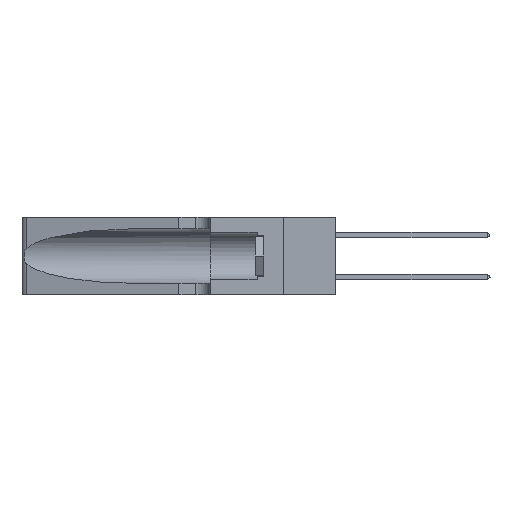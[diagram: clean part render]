
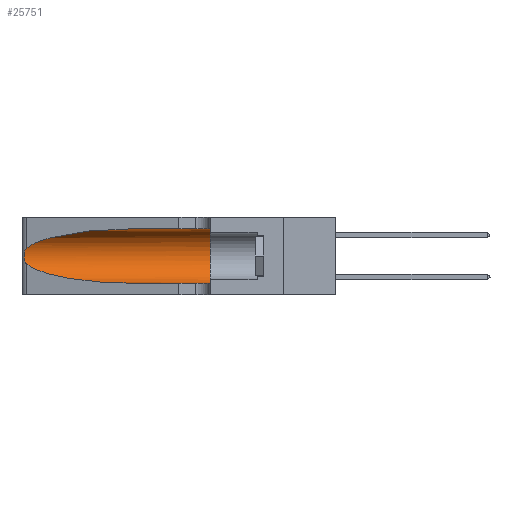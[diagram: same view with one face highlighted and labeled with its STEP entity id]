
A CAD part, left-side view. The second image highlights one B-rep face of the part: STEP entity #25751.
In plain terms, the highlighted cylindrical face has radius 3.308 mm (diameter 6.617 mm), a partial arc.
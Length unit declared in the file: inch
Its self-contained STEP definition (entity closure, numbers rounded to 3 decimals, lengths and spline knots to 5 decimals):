
#13 = EDGE_CURVE ( 'NONE', #23263, #21131, #15037, .T. ) ;
#1695 = CARTESIAN_POINT ( 'NONE',  ( 0.25487, 1.22718, 0.14631 ) ) ;
#2355 =( BOUNDED_CURVE ( )  B_SPLINE_CURVE ( 3, ( #11755, #7064, #9381, #26924 ),
 .UNSPECIFIED., .F., .F. ) 
 B_SPLINE_CURVE_WITH_KNOTS ( ( 4, 4 ),
 ( 1.5708, 2.84003 ),
 .UNSPECIFIED. ) 
 CURVE ( )  GEOMETRIC_REPRESENTATION_ITEM ( )  RATIONAL_B_SPLINE_CURVE ( ( 1., 0.87, 0.87, 1. ) ) 
 REPRESENTATION_ITEM ( '' )  );
#3142 = ORIENTED_EDGE ( 'NONE', *, *, #15293, .T. ) ;
#3192 = CARTESIAN_POINT ( 'NONE',  ( 0.25854, 1.2359, 0.20912 ) ) ;
#3483 = CARTESIAN_POINT ( 'NONE',  ( 0.25487, 1.22718, 0.22369 ) ) ;
#3599 = VECTOR ( 'NONE', #24083, 39.37008 ) ;
#3846 = CARTESIAN_POINT ( 'NONE',  ( 0.25555, 1.22993, 0.14849 ) ) ;
#4357 = EDGE_LOOP ( 'NONE', ( #8643, #21264, #3142, #8189, #12350, #24594 ) ) ;
#4475 = CARTESIAN_POINT ( 'NONE',  ( 0.1305, 0.35, 0.05475 ) ) ;
#4933 = CARTESIAN_POINT ( 'NONE',  ( 0.1305, 0.35, 0.185 ) ) ;
#5373 = CARTESIAN_POINT ( 'NONE',  ( 0.26018, 1.23835, 0.19895 ) ) ;
#5479 = CARTESIAN_POINT ( 'NONE',  ( 0.25789, 1.23486, 0.15765 ) ) ;
#6056 = CARTESIAN_POINT ( 'NONE',  ( 0.1305, 0.72297, 0.05475 ) ) ;
#6121 = EDGE_CURVE ( 'NONE', #26781, #21131, #25236, .T. ) ;
#6150 = CARTESIAN_POINT ( 'NONE',  ( 0.2373, 1.15595, 0.08982 ) ) ;
#6934 = EDGE_CURVE ( 'NONE', #13569, #14570, #2355, .T. ) ;
#7053 = EDGE_CURVE ( 'NONE', #14570, #12623, #9797, .T. ) ;
#7064 = CARTESIAN_POINT ( 'NONE',  ( 0.18966, 0.96281, 0.31525 ) ) ;
#7177 = VECTOR ( 'NONE', #27561, 39.37008 ) ;
#7535 = CARTESIAN_POINT ( 'NONE',  ( 0.26017, 1.23833, 0.17102 ) ) ;
#7549 = AXIS2_PLACEMENT_3D ( 'NONE', #26506, #23840, #15919 ) ;
#8189 = ORIENTED_EDGE ( 'NONE', *, *, #6121, .T. ) ;
#8643 = ORIENTED_EDGE ( 'NONE', *, *, #6934, .T. ) ;
#8868 = CARTESIAN_POINT ( 'NONE',  ( 0.1305, 1.61858, 0.05475 ) ) ;
#9381 = CARTESIAN_POINT ( 'NONE',  ( 0.2373, 1.15595, 0.28018 ) ) ;
#9797 = B_SPLINE_CURVE_WITH_KNOTS ( 'NONE', 3,
 ( #3483, #20782, #16224, #25213, #3192, #5373, #20591, #20500, #7535, #18415, #5479, #16697, #3846, #27856 ),
 .UNSPECIFIED., .F., .F.,
 ( 4, 2, 2, 2, 2, 2, 4 ),
 ( 0., 0.00027, 0.00053, 0.00107, 0.0016, 0.00187, 0.00214 ),
 .UNSPECIFIED. ) ;
#10388 = CARTESIAN_POINT ( 'NONE',  ( 0.1305, 0.72297, 0.05475 ) ) ;
#11755 = CARTESIAN_POINT ( 'NONE',  ( 0.1305, 0.72297, 0.31525 ) ) ;
#12350 = ORIENTED_EDGE ( 'NONE', *, *, #13, .F. ) ;
#12623 = VERTEX_POINT ( 'NONE', #17029 ) ;
#13258 = CYLINDRICAL_SURFACE ( 'NONE', #7549, 0.13025 ) ;
#13569 = VERTEX_POINT ( 'NONE', #23657 ) ;
#13755 = CARTESIAN_POINT ( 'NONE',  ( 0.25487, 1.22718, 0.22369 ) ) ;
#14315 = FACE_OUTER_BOUND ( 'NONE', #4357, .T. ) ;
#14570 = VERTEX_POINT ( 'NONE', #13755 ) ;
#14611 = LINE ( 'NONE', #25273, #7177 ) ;
#14883 = EDGE_CURVE ( 'NONE', #13569, #23263, #14611, .T. ) ;
#15037 = CIRCLE ( 'NONE', #24310, 0.13025 ) ;
#15293 = EDGE_CURVE ( 'NONE', #12623, #26781, #22816, .T. ) ;
#15919 = DIRECTION ( 'NONE',  ( 0., 0., -1. ) ) ;
#16224 = CARTESIAN_POINT ( 'NONE',  ( 0.25639, 1.23184, 0.21858 ) ) ;
#16697 = CARTESIAN_POINT ( 'NONE',  ( 0.25639, 1.23186, 0.15144 ) ) ;
#17029 = CARTESIAN_POINT ( 'NONE',  ( 0.25487, 1.22718, 0.14631 ) ) ;
#18179 = DIRECTION ( 'NONE',  ( 0., 0., 1. ) ) ;
#18415 = CARTESIAN_POINT ( 'NONE',  ( 0.25856, 1.23593, 0.16098 ) ) ;
#20068 = DIRECTION ( 'NONE',  ( 0., 1., 0. ) ) ;
#20500 = CARTESIAN_POINT ( 'NONE',  ( 0.26075, 1.23896, 0.178 ) ) ;
#20591 = CARTESIAN_POINT ( 'NONE',  ( 0.26075, 1.23896, 0.19203 ) ) ;
#20782 = CARTESIAN_POINT ( 'NONE',  ( 0.25555, 1.22994, 0.2215 ) ) ;
#21131 = VERTEX_POINT ( 'NONE', #4475 ) ;
#21264 = ORIENTED_EDGE ( 'NONE', *, *, #7053, .T. ) ;
#22117 = CARTESIAN_POINT ( 'NONE',  ( 0.1305, 0.35, 0.31525 ) ) ;
#22816 =( BOUNDED_CURVE ( )  B_SPLINE_CURVE ( 3, ( #1695, #6150, #27429, #6056 ),
 .UNSPECIFIED., .F., .F. ) 
 B_SPLINE_CURVE_WITH_KNOTS ( ( 4, 4 ),
 ( 3.44316, 4.71239 ),
 .UNSPECIFIED. ) 
 CURVE ( )  GEOMETRIC_REPRESENTATION_ITEM ( )  RATIONAL_B_SPLINE_CURVE ( ( 1., 0.87, 0.87, 1. ) ) 
 REPRESENTATION_ITEM ( '' )  );
#23263 = VERTEX_POINT ( 'NONE', #22117 ) ;
#23657 = CARTESIAN_POINT ( 'NONE',  ( 0.1305, 0.72297, 0.31525 ) ) ;
#23840 = DIRECTION ( 'NONE',  ( 0., -1., 0. ) ) ;
#24083 = DIRECTION ( 'NONE',  ( 0., -1., 0. ) ) ;
#24310 = AXIS2_PLACEMENT_3D ( 'NONE', #4933, #20068, #18179 ) ;
#24594 = ORIENTED_EDGE ( 'NONE', *, *, #14883, .F. ) ;
#25213 = CARTESIAN_POINT ( 'NONE',  ( 0.25787, 1.23484, 0.2124 ) ) ;
#25236 = LINE ( 'NONE', #8868, #3599 ) ;
#25273 = CARTESIAN_POINT ( 'NONE',  ( 0.1305, 1.61858, 0.31525 ) ) ;
#25751 = ADVANCED_FACE ( 'NONE', ( #14315 ), #13258, .F. ) ;
#26506 = CARTESIAN_POINT ( 'NONE',  ( 0.1305, 1.61858, 0.185 ) ) ;
#26781 = VERTEX_POINT ( 'NONE', #10388 ) ;
#26924 = CARTESIAN_POINT ( 'NONE',  ( 0.25487, 1.22718, 0.22369 ) ) ;
#27429 = CARTESIAN_POINT ( 'NONE',  ( 0.18966, 0.96281, 0.05475 ) ) ;
#27561 = DIRECTION ( 'NONE',  ( 0., -1., 0. ) ) ;
#27856 = CARTESIAN_POINT ( 'NONE',  ( 0.25487, 1.22718, 0.14631 ) ) ;
